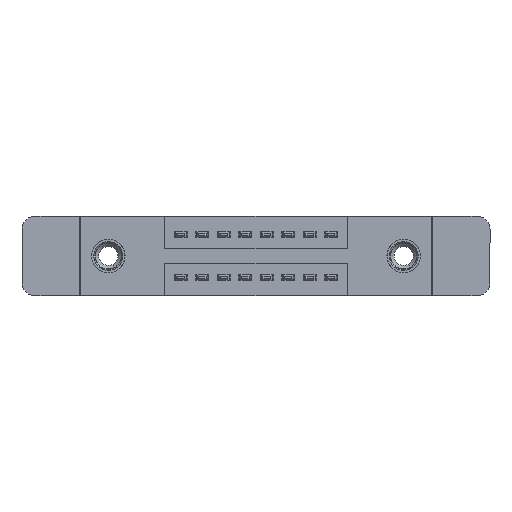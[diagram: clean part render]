
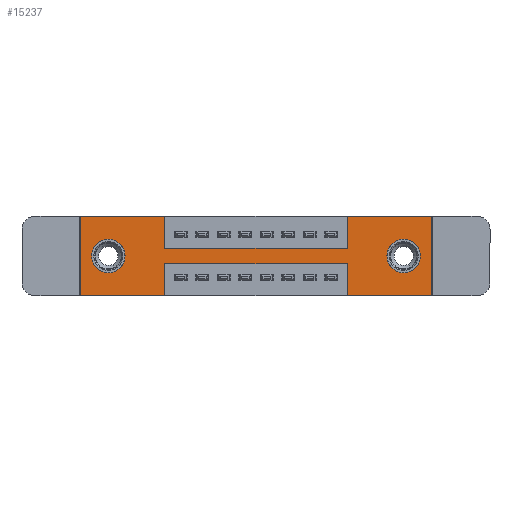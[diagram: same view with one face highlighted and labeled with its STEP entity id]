
A CAD part, front view. The second image highlights one B-rep face of the part: STEP entity #15237.
In plain terms, the highlighted planar face has unit normal (0, -1, 0).
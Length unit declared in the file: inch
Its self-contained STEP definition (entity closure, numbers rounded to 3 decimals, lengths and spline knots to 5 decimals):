
#222 = CARTESIAN_POINT ( 'NONE',  ( 0.13, 0., -0.107 ) ) ;
#334 = VERTEX_POINT ( 'NONE', #14188 ) ;
#450 = LINE ( 'NONE', #15262, #14792 ) ;
#515 = CARTESIAN_POINT ( 'NONE',  ( 0.13, 0., -0.185 ) ) ;
#676 = EDGE_LOOP ( 'NONE', ( #3127, #4094 ) ) ;
#747 = VERTEX_POINT ( 'NONE', #2223 ) ;
#779 = EDGE_CURVE ( 'NONE', #9846, #6474, #5042, .T. ) ;
#825 = DIRECTION ( 'NONE',  ( -1., 0., 0. ) ) ;
#1184 = CIRCLE ( 'NONE', #8089, 0.078 ) ;
#1278 = EDGE_LOOP ( 'NONE', ( #10023, #5539, #12420, #9782, #9553, #3623, #12286, #4423, #8274, #9787, #11831, #4869 ) ) ;
#1408 = VECTOR ( 'NONE', #10287, 39.37008 ) ;
#1474 = CARTESIAN_POINT ( 'NONE',  ( 1.2425, 0., -0.37 ) ) ;
#1571 = CARTESIAN_POINT ( 'NONE',  ( 1.505, 0., -0.185 ) ) ;
#1636 = CARTESIAN_POINT ( 'NONE',  ( 1.2425, 0., 0. ) ) ;
#1957 = CIRCLE ( 'NONE', #13227, 0.078 ) ;
#1969 = DIRECTION ( 'NONE',  ( 0., 0., -1. ) ) ;
#2223 = CARTESIAN_POINT ( 'NONE',  ( 0.3925, 0., -0.15 ) ) ;
#2423 = CARTESIAN_POINT ( 'NONE',  ( 0., 0., -0.37 ) ) ;
#2562 = VECTOR ( 'NONE', #8342, 39.37008 ) ;
#2572 = CARTESIAN_POINT ( 'NONE',  ( 0., 0., -0.37 ) ) ;
#2619 = DIRECTION ( 'NONE',  ( 1., 0., 0. ) ) ;
#2671 = LINE ( 'NONE', #15627, #15278 ) ;
#2677 = CARTESIAN_POINT ( 'NONE',  ( 0., 0., -0.37 ) ) ;
#3049 = EDGE_CURVE ( 'NONE', #5763, #3060, #12080, .T. ) ;
#3060 = VERTEX_POINT ( 'NONE', #2572 ) ;
#3122 = EDGE_CURVE ( 'NONE', #6474, #4228, #13027, .T. ) ;
#3126 = CARTESIAN_POINT ( 'NONE',  ( 0.3925, 0., 0. ) ) ;
#3127 = ORIENTED_EDGE ( 'NONE', *, *, #13160, .T. ) ;
#3357 = LINE ( 'NONE', #15069, #1408 ) ;
#3623 = ORIENTED_EDGE ( 'NONE', *, *, #6104, .F. ) ;
#3714 = ORIENTED_EDGE ( 'NONE', *, *, #8669, .T. ) ;
#3965 = LINE ( 'NONE', #3126, #12773 ) ;
#4094 = ORIENTED_EDGE ( 'NONE', *, *, #7195, .T. ) ;
#4228 = VERTEX_POINT ( 'NONE', #1474 ) ;
#4244 = CARTESIAN_POINT ( 'NONE',  ( 1.505, 0., -0.107 ) ) ;
#4257 = EDGE_CURVE ( 'NONE', #747, #12971, #15459, .T. ) ;
#4393 = CARTESIAN_POINT ( 'NONE',  ( 0., 0., -0.37 ) ) ;
#4423 = ORIENTED_EDGE ( 'NONE', *, *, #4257, .F. ) ;
#4538 = VERTEX_POINT ( 'NONE', #14643 ) ;
#4544 = DIRECTION ( 'NONE',  ( 1., 0., 0. ) ) ;
#4869 = ORIENTED_EDGE ( 'NONE', *, *, #3049, .F. ) ;
#4999 = DIRECTION ( 'NONE',  ( 0., 0., 1. ) ) ;
#5042 = LINE ( 'NONE', #10697, #2562 ) ;
#5220 = CARTESIAN_POINT ( 'NONE',  ( 1.2425, 0., -0.37 ) ) ;
#5429 = EDGE_CURVE ( 'NONE', #12971, #6134, #11436, .T. ) ;
#5539 = ORIENTED_EDGE ( 'NONE', *, *, #9978, .F. ) ;
#5548 = EDGE_CURVE ( 'NONE', #4538, #747, #3965, .T. ) ;
#5619 = CARTESIAN_POINT ( 'NONE',  ( 1.505, 0., -0.185 ) ) ;
#5763 = VERTEX_POINT ( 'NONE', #9170 ) ;
#5920 = DIRECTION ( 'NONE',  ( 0., 0., -1. ) ) ;
#6104 = EDGE_CURVE ( 'NONE', #6134, #9846, #13859, .T. ) ;
#6134 = VERTEX_POINT ( 'NONE', #9291 ) ;
#6198 = VERTEX_POINT ( 'NONE', #14208 ) ;
#6371 = DIRECTION ( 'NONE',  ( 0., 1., 0. ) ) ;
#6474 = VERTEX_POINT ( 'NONE', #12518 ) ;
#6646 = CARTESIAN_POINT ( 'NONE',  ( 0., 0., 0. ) ) ;
#6885 = EDGE_CURVE ( 'NONE', #3060, #12578, #450, .T. ) ;
#6901 = FACE_BOUND ( 'NONE', #9027, .T. ) ;
#6956 = EDGE_CURVE ( 'NONE', #6198, #5763, #3357, .T. ) ;
#7195 = EDGE_CURVE ( 'NONE', #8406, #8637, #15367, .T. ) ;
#7229 = CARTESIAN_POINT ( 'NONE',  ( 1.505, 0., -0.263 ) ) ;
#7439 = CARTESIAN_POINT ( 'NONE',  ( 1.2425, 0., -0.15 ) ) ;
#7779 = VECTOR ( 'NONE', #4544, 39.37008 ) ;
#8023 = FACE_BOUND ( 'NONE', #676, .T. ) ;
#8089 = AXIS2_PLACEMENT_3D ( 'NONE', #11801, #13011, #14210 ) ;
#8101 = CARTESIAN_POINT ( 'NONE',  ( 0., 0., 0. ) ) ;
#8121 = DIRECTION ( 'NONE',  ( 0., 0., -1. ) ) ;
#8274 = ORIENTED_EDGE ( 'NONE', *, *, #5548, .F. ) ;
#8342 = DIRECTION ( 'NONE',  ( 0., 0., -1. ) ) ;
#8406 = VERTEX_POINT ( 'NONE', #7229 ) ;
#8637 = VERTEX_POINT ( 'NONE', #4244 ) ;
#8669 = EDGE_CURVE ( 'NONE', #9030, #334, #11741, .T. ) ;
#8738 = EDGE_CURVE ( 'NONE', #334, #9030, #1184, .T. ) ;
#8776 = DIRECTION ( 'NONE',  ( 0., 0., -1. ) ) ;
#8884 = AXIS2_PLACEMENT_3D ( 'NONE', #5619, #15358, #5920 ) ;
#9027 = EDGE_LOOP ( 'NONE', ( #3714, #14155 ) ) ;
#9030 = VERTEX_POINT ( 'NONE', #222 ) ;
#9170 = CARTESIAN_POINT ( 'NONE',  ( 0.3925, 0., -0.37 ) ) ;
#9291 = CARTESIAN_POINT ( 'NONE',  ( 1.2425, 0., 0. ) ) ;
#9332 = CARTESIAN_POINT ( 'NONE',  ( 1.2425, 0., -0.22 ) ) ;
#9385 = AXIS2_PLACEMENT_3D ( 'NONE', #4393, #13003, #1969 ) ;
#9553 = ORIENTED_EDGE ( 'NONE', *, *, #779, .F. ) ;
#9782 = ORIENTED_EDGE ( 'NONE', *, *, #3122, .F. ) ;
#9787 = ORIENTED_EDGE ( 'NONE', *, *, #13248, .F. ) ;
#9846 = VERTEX_POINT ( 'NONE', #10493 ) ;
#9888 = VERTEX_POINT ( 'NONE', #9332 ) ;
#9978 = EDGE_CURVE ( 'NONE', #9888, #6198, #2671, .T. ) ;
#10023 = ORIENTED_EDGE ( 'NONE', *, *, #6956, .F. ) ;
#10186 = VECTOR ( 'NONE', #15038, 39.37008 ) ;
#10287 = DIRECTION ( 'NONE',  ( 0., 0., -1. ) ) ;
#10343 = DIRECTION ( 'NONE',  ( 0., 1., 0. ) ) ;
#10440 = DIRECTION ( 'NONE',  ( 0., 0., 1. ) ) ;
#10493 = CARTESIAN_POINT ( 'NONE',  ( 1.635, 0., 0. ) ) ;
#10507 = DIRECTION ( 'NONE',  ( 0., 0., 1. ) ) ;
#10697 = CARTESIAN_POINT ( 'NONE',  ( 1.635, 0., 0. ) ) ;
#10774 = LINE ( 'NONE', #6646, #11931 ) ;
#10921 = VECTOR ( 'NONE', #12747, 39.37008 ) ;
#11436 = LINE ( 'NONE', #1636, #11644 ) ;
#11467 = VECTOR ( 'NONE', #2619, 39.37008 ) ;
#11644 = VECTOR ( 'NONE', #4999, 39.37008 ) ;
#11741 = CIRCLE ( 'NONE', #15519, 0.078 ) ;
#11801 = CARTESIAN_POINT ( 'NONE',  ( 0.13, 0., -0.185 ) ) ;
#11831 = ORIENTED_EDGE ( 'NONE', *, *, #6885, .F. ) ;
#11931 = VECTOR ( 'NONE', #15200, 39.37008 ) ;
#12080 = LINE ( 'NONE', #2423, #14701 ) ;
#12286 = ORIENTED_EDGE ( 'NONE', *, *, #5429, .F. ) ;
#12420 = ORIENTED_EDGE ( 'NONE', *, *, #13199, .F. ) ;
#12518 = CARTESIAN_POINT ( 'NONE',  ( 1.635, 0., -0.37 ) ) ;
#12578 = VERTEX_POINT ( 'NONE', #14787 ) ;
#12747 = DIRECTION ( 'NONE',  ( -1., 0., 0. ) ) ;
#12773 = VECTOR ( 'NONE', #8121, 39.37008 ) ;
#12971 = VERTEX_POINT ( 'NONE', #7439 ) ;
#12993 = FACE_OUTER_BOUND ( 'NONE', #1278, .T. ) ;
#13003 = DIRECTION ( 'NONE',  ( 0., -1., 0. ) ) ;
#13011 = DIRECTION ( 'NONE',  ( 0., 1., 0. ) ) ;
#13027 = LINE ( 'NONE', #2677, #10921 ) ;
#13160 = EDGE_CURVE ( 'NONE', #8637, #8406, #1957, .T. ) ;
#13199 = EDGE_CURVE ( 'NONE', #4228, #9888, #14186, .T. ) ;
#13227 = AXIS2_PLACEMENT_3D ( 'NONE', #1571, #6371, #8776 ) ;
#13248 = EDGE_CURVE ( 'NONE', #12578, #4538, #10774, .T. ) ;
#13623 = CARTESIAN_POINT ( 'NONE',  ( 0.3925, 0., -0.15 ) ) ;
#13859 = LINE ( 'NONE', #8101, #7779 ) ;
#14038 = PLANE ( 'NONE',  #9385 ) ;
#14155 = ORIENTED_EDGE ( 'NONE', *, *, #8738, .T. ) ;
#14186 = LINE ( 'NONE', #5220, #10186 ) ;
#14188 = CARTESIAN_POINT ( 'NONE',  ( 0.13, 0., -0.263 ) ) ;
#14208 = CARTESIAN_POINT ( 'NONE',  ( 0.3925, 0., -0.22 ) ) ;
#14210 = DIRECTION ( 'NONE',  ( 0., 0., 1. ) ) ;
#14643 = CARTESIAN_POINT ( 'NONE',  ( 0.3925, 0., 0. ) ) ;
#14682 = DIRECTION ( 'NONE',  ( -1., 0., 0. ) ) ;
#14701 = VECTOR ( 'NONE', #14682, 39.37008 ) ;
#14787 = CARTESIAN_POINT ( 'NONE',  ( 0., 0., 0. ) ) ;
#14792 = VECTOR ( 'NONE', #10440, 39.37008 ) ;
#15038 = DIRECTION ( 'NONE',  ( 0., 0., 1. ) ) ;
#15069 = CARTESIAN_POINT ( 'NONE',  ( 0.3925, 0., -0.37 ) ) ;
#15200 = DIRECTION ( 'NONE',  ( 1., 0., 0. ) ) ;
#15237 = ADVANCED_FACE ( 'NONE', ( #8023, #6901, #12993 ), #14038, .T. ) ;
#15262 = CARTESIAN_POINT ( 'NONE',  ( 0., 0., 0. ) ) ;
#15278 = VECTOR ( 'NONE', #825, 39.37008 ) ;
#15358 = DIRECTION ( 'NONE',  ( 0., 1., 0. ) ) ;
#15367 = CIRCLE ( 'NONE', #8884, 0.078 ) ;
#15459 = LINE ( 'NONE', #13623, #11467 ) ;
#15519 = AXIS2_PLACEMENT_3D ( 'NONE', #515, #10343, #10507 ) ;
#15627 = CARTESIAN_POINT ( 'NONE',  ( 0.3925, 0., -0.22 ) ) ;
